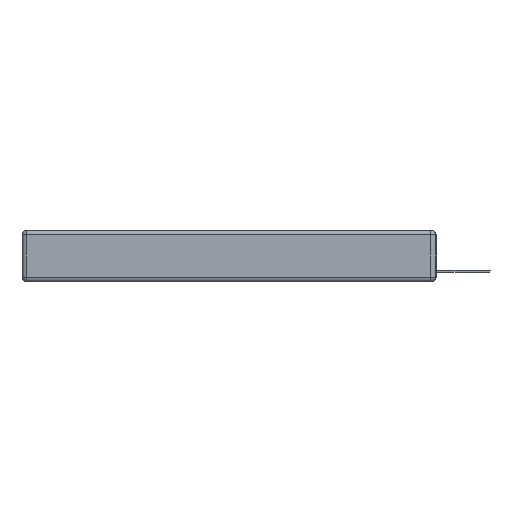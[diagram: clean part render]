
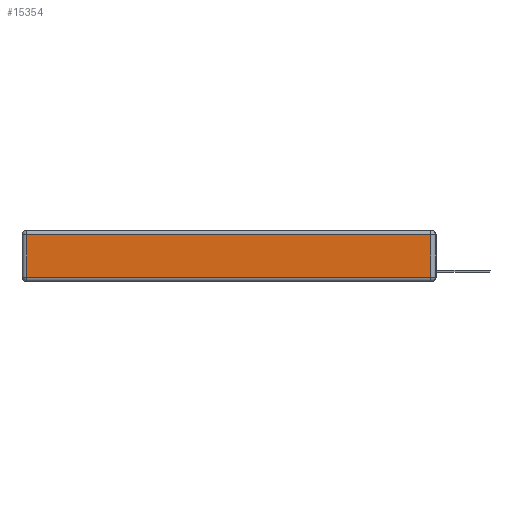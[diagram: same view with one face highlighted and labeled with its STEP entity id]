
A CAD part, left-side view. The second image highlights one B-rep face of the part: STEP entity #15354.
In plain terms, the highlighted planar face has unit normal (-1, 0, 0).
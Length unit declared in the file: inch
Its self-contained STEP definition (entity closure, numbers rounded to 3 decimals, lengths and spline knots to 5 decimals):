
#956 = DIRECTION ( 'NONE',  ( 0., 0., 1. ) ) ;
#1464 = VERTEX_POINT ( 'NONE', #11106 ) ;
#1569 = CARTESIAN_POINT ( 'NONE',  ( 0., 0.03, -0.343 ) ) ;
#1666 = CARTESIAN_POINT ( 'NONE',  ( 0., 2.75, -0.03 ) ) ;
#2430 = VERTEX_POINT ( 'NONE', #10614 ) ;
#2467 = EDGE_LOOP ( 'NONE', ( #8942, #3496, #11079, #4335 ) ) ;
#2626 = DIRECTION ( 'NONE',  ( 0., 0., 1. ) ) ;
#2700 = EDGE_CURVE ( 'NONE', #13944, #2430, #8830, .T. ) ;
#2859 = CARTESIAN_POINT ( 'NONE',  ( 0., 0., -0.313 ) ) ;
#3146 = AXIS2_PLACEMENT_3D ( 'NONE', #6945, #13031, #956 ) ;
#3496 = ORIENTED_EDGE ( 'NONE', *, *, #2700, .T. ) ;
#3591 = CARTESIAN_POINT ( 'NONE',  ( 0., 2.72, -0.313 ) ) ;
#3654 = CARTESIAN_POINT ( 'NONE',  ( 0., 0.03, -0.313 ) ) ;
#3779 = VECTOR ( 'NONE', #2626, 39.37008 ) ;
#3829 = LINE ( 'NONE', #13948, #5080 ) ;
#4335 = ORIENTED_EDGE ( 'NONE', *, *, #4554, .T. ) ;
#4554 = EDGE_CURVE ( 'NONE', #1464, #6943, #3829, .T. ) ;
#5080 = VECTOR ( 'NONE', #12480, 39.37008 ) ;
#5137 = LINE ( 'NONE', #2859, #9261 ) ;
#5547 = VECTOR ( 'NONE', #7799, 39.37008 ) ;
#6943 = VERTEX_POINT ( 'NONE', #3591 ) ;
#6945 = CARTESIAN_POINT ( 'NONE',  ( 0., 0., -0.343 ) ) ;
#7194 = EDGE_CURVE ( 'NONE', #6943, #13944, #5137, .T. ) ;
#7799 = DIRECTION ( 'NONE',  ( 0., 1., 0. ) ) ;
#8294 = PLANE ( 'NONE',  #3146 ) ;
#8830 = LINE ( 'NONE', #1569, #3779 ) ;
#8942 = ORIENTED_EDGE ( 'NONE', *, *, #7194, .T. ) ;
#9261 = VECTOR ( 'NONE', #15085, 39.37008 ) ;
#10614 = CARTESIAN_POINT ( 'NONE',  ( 0., 0.03, -0.03 ) ) ;
#11079 = ORIENTED_EDGE ( 'NONE', *, *, #11801, .T. ) ;
#11106 = CARTESIAN_POINT ( 'NONE',  ( 0., 2.72, -0.03 ) ) ;
#11801 = EDGE_CURVE ( 'NONE', #2430, #1464, #15358, .T. ) ;
#12480 = DIRECTION ( 'NONE',  ( 0., 0., -1. ) ) ;
#13031 = DIRECTION ( 'NONE',  ( -1., 0., 0. ) ) ;
#13598 = FACE_OUTER_BOUND ( 'NONE', #2467, .T. ) ;
#13944 = VERTEX_POINT ( 'NONE', #3654 ) ;
#13948 = CARTESIAN_POINT ( 'NONE',  ( 0., 2.72, -0.343 ) ) ;
#15085 = DIRECTION ( 'NONE',  ( 0., -1., 0. ) ) ;
#15354 = ADVANCED_FACE ( 'NONE', ( #13598 ), #8294, .T. ) ;
#15358 = LINE ( 'NONE', #1666, #5547 ) ;
